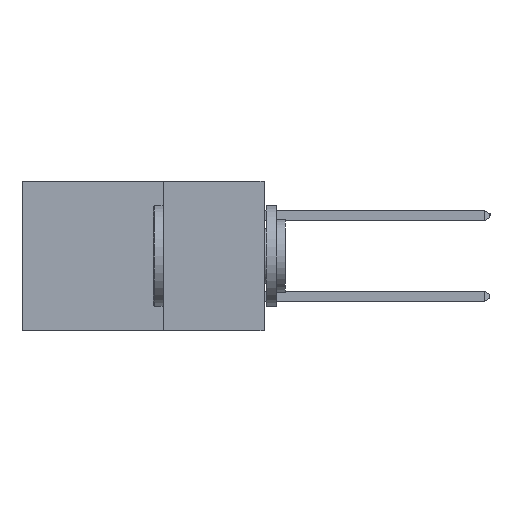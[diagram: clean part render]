
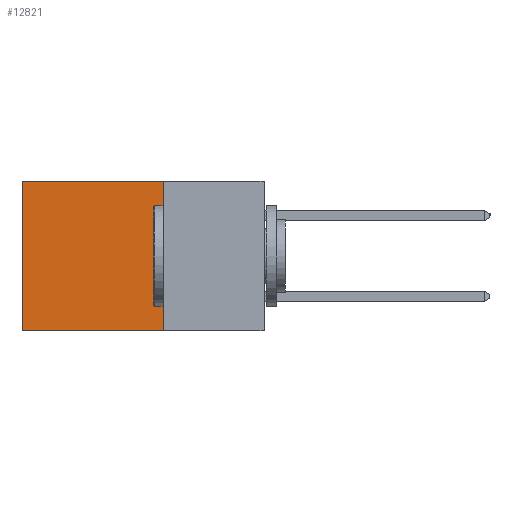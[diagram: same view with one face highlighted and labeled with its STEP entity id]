
A CAD part, left-side view. The second image highlights one B-rep face of the part: STEP entity #12821.
In plain terms, the highlighted planar face has unit normal (-1, 0, 0).
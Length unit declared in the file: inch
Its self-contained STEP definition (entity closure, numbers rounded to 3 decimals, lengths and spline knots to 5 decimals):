
#757 = VECTOR ( 'NONE', #7547, 39.37008 ) ;
#791 = DIRECTION ( 'NONE',  ( 1., 0., 0. ) ) ;
#1079 = VECTOR ( 'NONE', #11481, 39.37008 ) ;
#1975 = CARTESIAN_POINT ( 'NONE',  ( 0.2615, 0.25, 0. ) ) ;
#2142 = FACE_OUTER_BOUND ( 'NONE', #6598, .T. ) ;
#2151 = DIRECTION ( 'NONE',  ( 0., 1., 0. ) ) ;
#2369 = LINE ( 'NONE', #14787, #1079 ) ;
#2397 = EDGE_CURVE ( 'NONE', #14744, #3630, #4562, .T. ) ;
#2995 = ORIENTED_EDGE ( 'NONE', *, *, #2397, .F. ) ;
#3429 = VECTOR ( 'NONE', #2151, 39.37008 ) ;
#3630 = VERTEX_POINT ( 'NONE', #10829 ) ;
#4178 = PLANE ( 'NONE',  #11167 ) ;
#4336 = DIRECTION ( 'NONE',  ( 0., 0., -1. ) ) ;
#4562 = LINE ( 'NONE', #5611, #7676 ) ;
#5506 = VERTEX_POINT ( 'NONE', #1975 ) ;
#5611 = CARTESIAN_POINT ( 'NONE',  ( 0.2615, 0.25, -0.37 ) ) ;
#6201 = LINE ( 'NONE', #6343, #757 ) ;
#6257 = VERTEX_POINT ( 'NONE', #7205 ) ;
#6343 = CARTESIAN_POINT ( 'NONE',  ( 0.2615, 0.6, -0.37 ) ) ;
#6598 = EDGE_LOOP ( 'NONE', ( #6635, #2995, #9897, #13370 ) ) ;
#6635 = ORIENTED_EDGE ( 'NONE', *, *, #7228, .T. ) ;
#7205 = CARTESIAN_POINT ( 'NONE',  ( 0.2615, 0.6, 0. ) ) ;
#7228 = EDGE_CURVE ( 'NONE', #6257, #3630, #6201, .T. ) ;
#7547 = DIRECTION ( 'NONE',  ( 0., 0., -1. ) ) ;
#7676 = VECTOR ( 'NONE', #12461, 39.37008 ) ;
#8282 = EDGE_CURVE ( 'NONE', #5506, #6257, #10216, .T. ) ;
#9018 = CARTESIAN_POINT ( 'NONE',  ( 0.2615, 0.25, 0. ) ) ;
#9897 = ORIENTED_EDGE ( 'NONE', *, *, #12923, .F. ) ;
#10216 = LINE ( 'NONE', #9018, #3429 ) ;
#10829 = CARTESIAN_POINT ( 'NONE',  ( 0.2615, 0.6, -0.37 ) ) ;
#11167 = AXIS2_PLACEMENT_3D ( 'NONE', #12224, #791, #4336 ) ;
#11481 = DIRECTION ( 'NONE',  ( 0., 0., -1. ) ) ;
#12224 = CARTESIAN_POINT ( 'NONE',  ( 0.2615, 0.25, -0.37 ) ) ;
#12461 = DIRECTION ( 'NONE',  ( 0., 1., 0. ) ) ;
#12821 = ADVANCED_FACE ( 'NONE', ( #2142 ), #4178, .F. ) ;
#12923 = EDGE_CURVE ( 'NONE', #5506, #14744, #2369, .T. ) ;
#13281 = CARTESIAN_POINT ( 'NONE',  ( 0.2615, 0.25, -0.37 ) ) ;
#13370 = ORIENTED_EDGE ( 'NONE', *, *, #8282, .T. ) ;
#14744 = VERTEX_POINT ( 'NONE', #13281 ) ;
#14787 = CARTESIAN_POINT ( 'NONE',  ( 0.2615, 0.25, -0.37 ) ) ;
